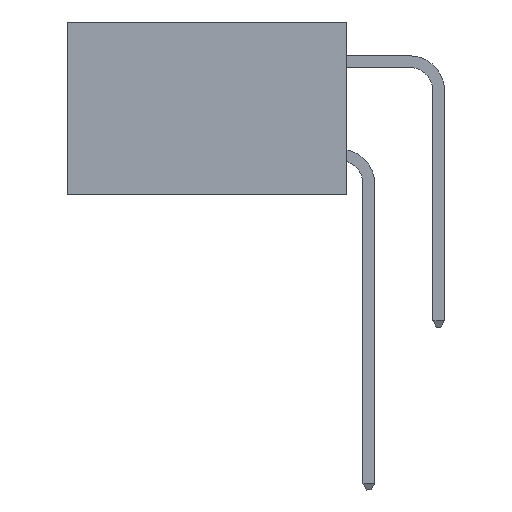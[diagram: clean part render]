
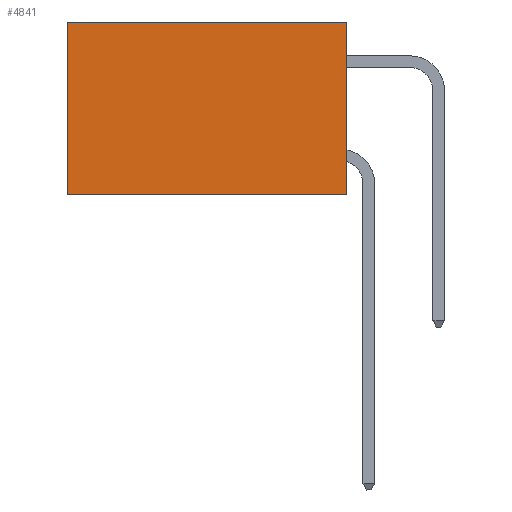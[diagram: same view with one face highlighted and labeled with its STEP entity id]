
A CAD part, left-side view. The second image highlights one B-rep face of the part: STEP entity #4841.
In plain terms, the highlighted planar face has unit normal (-1, 0, 0).
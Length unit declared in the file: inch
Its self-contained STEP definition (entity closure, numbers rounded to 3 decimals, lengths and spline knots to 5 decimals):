
#285 = FACE_OUTER_BOUND ( 'NONE', #2454, .T. ) ;
#1431 = DIRECTION ( 'NONE',  ( 0., 0., -1. ) ) ;
#2396 = LINE ( 'NONE', #7810, #17920 ) ;
#2454 = EDGE_LOOP ( 'NONE', ( #3851, #3346, #3233, #16813 ) ) ;
#3233 = ORIENTED_EDGE ( 'NONE', *, *, #10994, .F. ) ;
#3346 = ORIENTED_EDGE ( 'NONE', *, *, #13933, .F. ) ;
#3851 = ORIENTED_EDGE ( 'NONE', *, *, #16162, .T. ) ;
#4841 = ADVANCED_FACE ( 'NONE', ( #285 ), #6184, .F. ) ;
#5688 = VERTEX_POINT ( 'NONE', #17374 ) ;
#6184 = PLANE ( 'NONE',  #13723 ) ;
#7338 = VECTOR ( 'NONE', #7540, 39.37008 ) ;
#7540 = DIRECTION ( 'NONE',  ( 0., 1., 0. ) ) ;
#7810 = CARTESIAN_POINT ( 'NONE',  ( 0.2875, 0., 0. ) ) ;
#8659 = VERTEX_POINT ( 'NONE', #14983 ) ;
#9272 = CARTESIAN_POINT ( 'NONE',  ( 0.2875, 0., 0. ) ) ;
#9818 = DIRECTION ( 'NONE',  ( 0., 0., -1. ) ) ;
#9889 = DIRECTION ( 'NONE',  ( 0., 0., -1. ) ) ;
#10848 = DIRECTION ( 'NONE',  ( 1., 0., 0. ) ) ;
#10994 = EDGE_CURVE ( 'NONE', #14941, #8659, #11039, .T. ) ;
#11039 = LINE ( 'NONE', #17461, #14705 ) ;
#11718 = CARTESIAN_POINT ( 'NONE',  ( 0.2875, 0., 0. ) ) ;
#12620 = EDGE_CURVE ( 'NONE', #14941, #5688, #2396, .T. ) ;
#13723 = AXIS2_PLACEMENT_3D ( 'NONE', #9272, #10848, #1431 ) ;
#13933 = EDGE_CURVE ( 'NONE', #8659, #15591, #19032, .T. ) ;
#14705 = VECTOR ( 'NONE', #9818, 39.37008 ) ;
#14941 = VERTEX_POINT ( 'NONE', #11718 ) ;
#14983 = CARTESIAN_POINT ( 'NONE',  ( 0.2875, 0., -0.37 ) ) ;
#15591 = VERTEX_POINT ( 'NONE', #19222 ) ;
#16162 = EDGE_CURVE ( 'NONE', #5688, #15591, #18216, .T. ) ;
#16641 = VECTOR ( 'NONE', #9889, 39.37008 ) ;
#16771 = CARTESIAN_POINT ( 'NONE',  ( 0.2875, 0., -0.37 ) ) ;
#16813 = ORIENTED_EDGE ( 'NONE', *, *, #12620, .T. ) ;
#17374 = CARTESIAN_POINT ( 'NONE',  ( 0.2875, 0.6, 0. ) ) ;
#17461 = CARTESIAN_POINT ( 'NONE',  ( 0.2875, 0., 0. ) ) ;
#17920 = VECTOR ( 'NONE', #19963, 39.37008 ) ;
#18216 = LINE ( 'NONE', #19009, #16641 ) ;
#19009 = CARTESIAN_POINT ( 'NONE',  ( 0.2875, 0.6, 0. ) ) ;
#19032 = LINE ( 'NONE', #16771, #7338 ) ;
#19222 = CARTESIAN_POINT ( 'NONE',  ( 0.2875, 0.6, -0.37 ) ) ;
#19963 = DIRECTION ( 'NONE',  ( 0., 1., 0. ) ) ;
